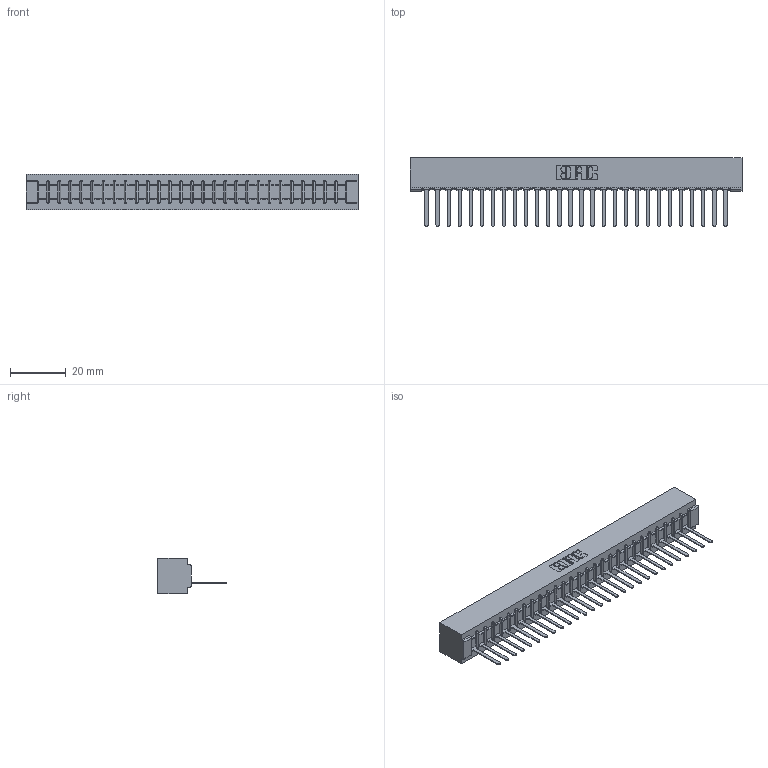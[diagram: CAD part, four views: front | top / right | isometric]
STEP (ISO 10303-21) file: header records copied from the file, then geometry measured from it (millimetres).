
FILE_DESCRIPTION (( 'STEP AP203' ), '1' );
FILE_NAME ('357-028-541-101.STEP', '2018-08-09T06:02:51', ( '' ), ( '' ), 'SwSTEP 2.0', 'SolidWorks 2016', '' );
FILE_SCHEMA (( 'CONFIG_CONTROL_DESIGN' ));
Length unit declared in the file: inch
Products named in the file (3): 307 Part_No Mounting Lugs; 307-290-002_541; 357-028-541-101
Assembly tree (29 placements, depth 2):
  357-028-541-101
    307 Part_No Mounting Lugs
    307-290-002_541  x28
Bounding box: 118.82 x 24.59 x 12.7 mm (x, y, z)
Volume: 13247.8 mm3; surface area: 17208.9 mm2
Topology: 29 solids, 29 shells, 2211 faces, 6795 edges, 4450 vertices
Faces by surface type: plane 1326, cylinder 827, sphere 58
Entity records: 26170 total; most frequent: CARTESIAN_POINT 4412, ORIENTED_EDGE 4402, DIRECTION 4291, EDGE_CURVE 2201, LINE 1681, VECTOR 1681, VERTEX_POINT 1426, AXIS2_PLACEMENT_3D 1305
